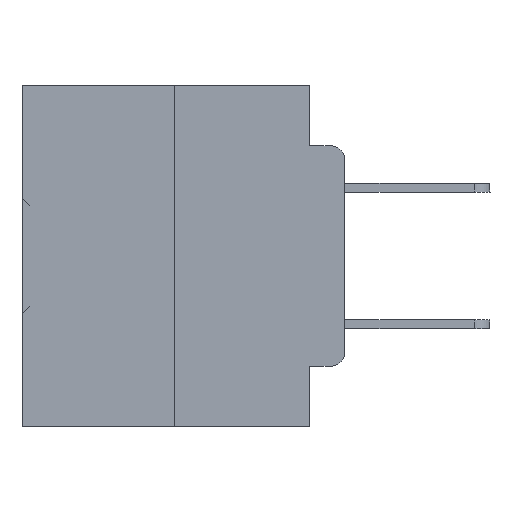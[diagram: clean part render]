
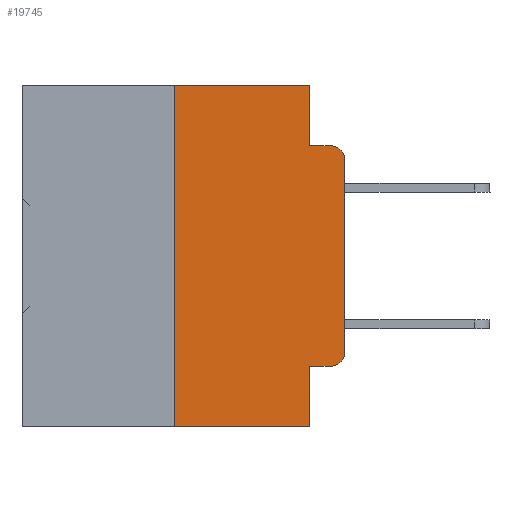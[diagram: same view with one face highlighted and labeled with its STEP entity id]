
A CAD part, left-side view. The second image highlights one B-rep face of the part: STEP entity #19745.
In plain terms, the highlighted planar face has unit normal (-1, 0, 0).
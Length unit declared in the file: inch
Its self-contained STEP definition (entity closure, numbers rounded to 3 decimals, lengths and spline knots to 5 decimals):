
#166 = LINE ( 'NONE', #35856, #25470 ) ;
#725 = LINE ( 'NONE', #6774, #9069 ) ;
#790 = DIRECTION ( 'NONE',  ( 0., 0., -1. ) ) ;
#998 = LINE ( 'NONE', #22629, #27339 ) ;
#1298 = CARTESIAN_POINT ( 'NONE',  ( 0., 0.051, 0. ) ) ;
#1537 = CARTESIAN_POINT ( 'NONE',  ( 0., 0.02, -0.0885 ) ) ;
#1583 = CARTESIAN_POINT ( 'NONE',  ( 0., 0.473, 0. ) ) ;
#1795 = EDGE_CURVE ( 'NONE', #7289, #30359, #13188, .T. ) ;
#2657 = CARTESIAN_POINT ( 'NONE',  ( 0., 0.25, 0. ) ) ;
#2856 = CARTESIAN_POINT ( 'NONE',  ( 0., 0.02, -0.1085 ) ) ;
#3254 = CARTESIAN_POINT ( 'NONE',  ( 0., 0.051, -0.5 ) ) ;
#3372 = ORIENTED_EDGE ( 'NONE', *, *, #22120, .F. ) ;
#4142 = CARTESIAN_POINT ( 'NONE',  ( 0., 0.473, 0. ) ) ;
#4235 = EDGE_CURVE ( 'NONE', #38164, #34864, #20171, .T. ) ;
#4289 = DIRECTION ( 'NONE',  ( 0., 0., -1. ) ) ;
#4729 = DIRECTION ( 'NONE',  ( 0., 0., -1. ) ) ;
#4775 = EDGE_CURVE ( 'NONE', #23545, #38164, #13745, .T. ) ;
#4990 = CARTESIAN_POINT ( 'NONE',  ( 0., 0.051, -0.4115 ) ) ;
#5180 = VERTEX_POINT ( 'NONE', #13848 ) ;
#5346 = VERTEX_POINT ( 'NONE', #32554 ) ;
#6473 = EDGE_CURVE ( 'NONE', #7987, #5180, #998, .T. ) ;
#6774 = CARTESIAN_POINT ( 'NONE',  ( 0., 0.473, -0.5 ) ) ;
#6949 = CARTESIAN_POINT ( 'NONE',  ( 0., 0., -0.1085 ) ) ;
#7289 = VERTEX_POINT ( 'NONE', #6949 ) ;
#7891 = ORIENTED_EDGE ( 'NONE', *, *, #9420, .F. ) ;
#7987 = VERTEX_POINT ( 'NONE', #35176 ) ;
#8873 = VECTOR ( 'NONE', #11009, 39.37008 ) ;
#9069 = VECTOR ( 'NONE', #21199, 39.37008 ) ;
#9420 = EDGE_CURVE ( 'NONE', #5180, #30359, #11196, .T. ) ;
#11009 = DIRECTION ( 'NONE',  ( 0., -1., 0. ) ) ;
#11196 = LINE ( 'NONE', #29733, #8873 ) ;
#11228 = DIRECTION ( 'NONE',  ( -1., 0., 0. ) ) ;
#11547 = EDGE_LOOP ( 'NONE', ( #32999, #32943, #7891, #14584, #27954, #32091, #21718, #3372, #21522, #27462 ) ) ;
#13188 = CIRCLE ( 'NONE', #23776, 0.02 ) ;
#13745 = LINE ( 'NONE', #16858, #28317 ) ;
#13848 = CARTESIAN_POINT ( 'NONE',  ( 0., 0.051, -0.0885 ) ) ;
#14584 = ORIENTED_EDGE ( 'NONE', *, *, #6473, .F. ) ;
#16628 = PLANE ( 'NONE',  #19494 ) ;
#16858 = CARTESIAN_POINT ( 'NONE',  ( 0., 0.051, -0.4115 ) ) ;
#17952 = CARTESIAN_POINT ( 'NONE',  ( 0., 0.02, -0.3915 ) ) ;
#18922 = AXIS2_PLACEMENT_3D ( 'NONE', #17952, #30062, #790 ) ;
#19109 = DIRECTION ( 'NONE',  ( 0., -1., 0. ) ) ;
#19494 = AXIS2_PLACEMENT_3D ( 'NONE', #4142, #27760, #4729 ) ;
#19745 = ADVANCED_FACE ( 'NONE', ( #31048 ), #16628, .F. ) ;
#20171 = CIRCLE ( 'NONE', #18922, 0.02 ) ;
#21199 = DIRECTION ( 'NONE',  ( 0., -1., 0. ) ) ;
#21522 = ORIENTED_EDGE ( 'NONE', *, *, #4775, .T. ) ;
#21624 = EDGE_CURVE ( 'NONE', #31797, #7987, #25175, .T. ) ;
#21718 = ORIENTED_EDGE ( 'NONE', *, *, #33798, .T. ) ;
#22120 = EDGE_CURVE ( 'NONE', #23545, #30496, #30563, .T. ) ;
#22535 = DIRECTION ( 'NONE',  ( 0., 0., -1. ) ) ;
#22629 = CARTESIAN_POINT ( 'NONE',  ( 0., 0.051, 0. ) ) ;
#23545 = VERTEX_POINT ( 'NONE', #4990 ) ;
#23575 = CARTESIAN_POINT ( 'NONE',  ( 0., 0.25, 0. ) ) ;
#23758 = VECTOR ( 'NONE', #19109, 39.37008 ) ;
#23776 = AXIS2_PLACEMENT_3D ( 'NONE', #2856, #11228, #34842 ) ;
#23814 = VECTOR ( 'NONE', #22535, 39.37008 ) ;
#25175 = LINE ( 'NONE', #1583, #23758 ) ;
#25470 = VECTOR ( 'NONE', #30000, 39.37008 ) ;
#26135 = VECTOR ( 'NONE', #26438, 39.37008 ) ;
#26224 = LINE ( 'NONE', #2657, #26135 ) ;
#26438 = DIRECTION ( 'NONE',  ( 0., 0., 1. ) ) ;
#27339 = VECTOR ( 'NONE', #4289, 39.37008 ) ;
#27462 = ORIENTED_EDGE ( 'NONE', *, *, #4235, .T. ) ;
#27760 = DIRECTION ( 'NONE',  ( 1., 0., 0. ) ) ;
#27954 = ORIENTED_EDGE ( 'NONE', *, *, #21624, .F. ) ;
#28317 = VECTOR ( 'NONE', #37531, 39.37008 ) ;
#28706 = EDGE_CURVE ( 'NONE', #34864, #7289, #166, .T. ) ;
#28993 = EDGE_CURVE ( 'NONE', #5346, #31797, #26224, .T. ) ;
#29733 = CARTESIAN_POINT ( 'NONE',  ( 0., 0.051, -0.0885 ) ) ;
#30000 = DIRECTION ( 'NONE',  ( 0., 0., 1. ) ) ;
#30062 = DIRECTION ( 'NONE',  ( -1., 0., 0. ) ) ;
#30359 = VERTEX_POINT ( 'NONE', #1537 ) ;
#30496 = VERTEX_POINT ( 'NONE', #3254 ) ;
#30563 = LINE ( 'NONE', #1298, #23814 ) ;
#31048 = FACE_OUTER_BOUND ( 'NONE', #11547, .T. ) ;
#31797 = VERTEX_POINT ( 'NONE', #23575 ) ;
#32091 = ORIENTED_EDGE ( 'NONE', *, *, #28993, .F. ) ;
#32554 = CARTESIAN_POINT ( 'NONE',  ( 0., 0.25, -0.5 ) ) ;
#32943 = ORIENTED_EDGE ( 'NONE', *, *, #1795, .T. ) ;
#32999 = ORIENTED_EDGE ( 'NONE', *, *, #28706, .T. ) ;
#33798 = EDGE_CURVE ( 'NONE', #5346, #30496, #725, .T. ) ;
#34842 = DIRECTION ( 'NONE',  ( 0., 0., -1. ) ) ;
#34864 = VERTEX_POINT ( 'NONE', #36596 ) ;
#35176 = CARTESIAN_POINT ( 'NONE',  ( 0., 0.051, 0. ) ) ;
#35856 = CARTESIAN_POINT ( 'NONE',  ( 0., 0., 0. ) ) ;
#36596 = CARTESIAN_POINT ( 'NONE',  ( 0., 0., -0.3915 ) ) ;
#36609 = CARTESIAN_POINT ( 'NONE',  ( 0., 0.02, -0.4115 ) ) ;
#37531 = DIRECTION ( 'NONE',  ( 0., -1., 0. ) ) ;
#38164 = VERTEX_POINT ( 'NONE', #36609 ) ;
